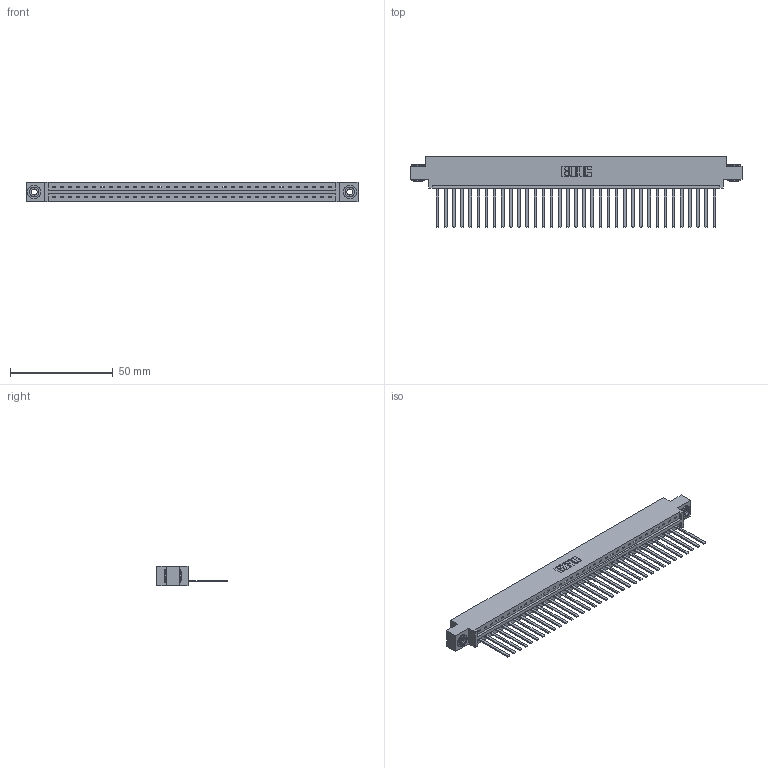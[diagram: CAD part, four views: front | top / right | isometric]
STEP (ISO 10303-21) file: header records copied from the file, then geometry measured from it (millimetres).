
FILE_DESCRIPTION (( 'STEP AP203' ), '1' );
FILE_NAME ('387-035-544-603.STEP', '2019-10-04T12:39:15', ( '' ), ( '' ), 'SwSTEP 2.0', 'SolidWorks 2016', '' );
FILE_SCHEMA (( 'CONFIG_CONTROL_DESIGN' ));
Length unit declared in the file: inch
Products named in the file (4): 345-250-002_345-250-002-102; 345-292-001_345-293-144; 337 Part_0.170 Offset - 0.156 Dia-TH; 387-035-544-603
Assembly tree (38 placements, depth 2):
  387-035-544-603
    337 Part_0.170 Offset - 0.156 Dia-TH
    345-292-001_345-293-144  x35
    345-250-002_345-250-002-102  x2
Bounding box: 161.7 x 34.3 x 9.4 mm (x, y, z)
Volume: 17025.3 mm3; surface area: 19216.8 mm2
Topology: 38 solids, 38 shells, 2116 faces, 6349 edges, 4182 vertices
Faces by surface type: plane 1554, cylinder 554, cone 8
Entity records: 27520 total; most frequent: CARTESIAN_POINT 4770, ORIENTED_EDGE 4734, DIRECTION 4059, EDGE_CURVE 2367, VECTOR 2219, LINE 2219, VERTEX_POINT 1574, AXIS2_PLACEMENT_3D 920
